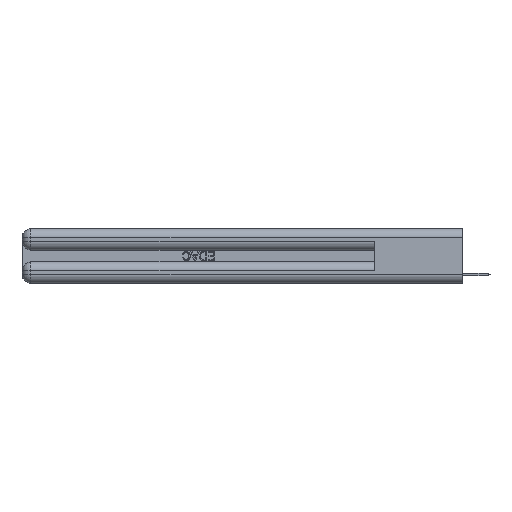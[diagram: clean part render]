
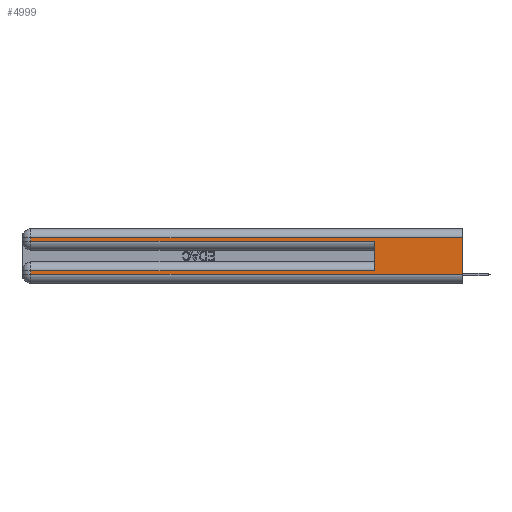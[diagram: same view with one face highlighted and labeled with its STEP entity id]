
A CAD part, left-side view. The second image highlights one B-rep face of the part: STEP entity #4999.
In plain terms, the highlighted planar face has unit normal (-1, 0, 0).
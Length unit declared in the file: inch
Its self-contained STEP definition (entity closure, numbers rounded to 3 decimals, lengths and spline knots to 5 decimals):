
#286 = EDGE_CURVE ( 'NONE', #21872, #2291, #27321, .T. ) ;
#1139 = CARTESIAN_POINT ( 'NONE',  ( 0., 0.6, 0.145 ) ) ;
#1155 = VECTOR ( 'NONE', #3932, 39.37008 ) ;
#2291 = VERTEX_POINT ( 'NONE', #21210 ) ;
#3072 = CARTESIAN_POINT ( 'NONE',  ( 0., 2.94, 0.06 ) ) ;
#3932 = DIRECTION ( 'NONE',  ( 0., -1., 0. ) ) ;
#4457 = FACE_OUTER_BOUND ( 'NONE', #8064, .T. ) ;
#4999 = ADVANCED_FACE ( 'NONE', ( #4457 ), #14202, .F. ) ;
#5020 = LINE ( 'NONE', #7411, #5801 ) ;
#5404 = VERTEX_POINT ( 'NONE', #13728 ) ;
#5482 = ORIENTED_EDGE ( 'NONE', *, *, #11655, .T. ) ;
#5722 = CARTESIAN_POINT ( 'NONE',  ( 0., 2.94, 0.285 ) ) ;
#5801 = VECTOR ( 'NONE', #27592, 39.37008 ) ;
#5935 = VECTOR ( 'NONE', #7160, 39.37008 ) ;
#6529 = ORIENTED_EDGE ( 'NONE', *, *, #286, .T. ) ;
#6652 = VERTEX_POINT ( 'NONE', #5722 ) ;
#7160 = DIRECTION ( 'NONE',  ( 0., 0., -1. ) ) ;
#7411 = CARTESIAN_POINT ( 'NONE',  ( 0., 0., 0.37 ) ) ;
#7462 = VECTOR ( 'NONE', #11444, 39.37008 ) ;
#7472 = VERTEX_POINT ( 'NONE', #28420 ) ;
#8064 = EDGE_LOOP ( 'NONE', ( #13339, #16782, #17089, #28735, #31666, #5482, #27351, #6529 ) ) ;
#8271 = EDGE_CURVE ( 'NONE', #6652, #22296, #17058, .T. ) ;
#9821 = CARTESIAN_POINT ( 'NONE',  ( 0., 0.6, 0.285 ) ) ;
#10339 = LINE ( 'NONE', #24592, #5935 ) ;
#11444 = DIRECTION ( 'NONE',  ( 0., 0., -1. ) ) ;
#11655 = EDGE_CURVE ( 'NONE', #20046, #5404, #31881, .T. ) ;
#12209 = LINE ( 'NONE', #31025, #7462 ) ;
#13339 = ORIENTED_EDGE ( 'NONE', *, *, #27402, .F. ) ;
#13593 = DIRECTION ( 'NONE',  ( 1., 0., 0. ) ) ;
#13728 = CARTESIAN_POINT ( 'NONE',  ( 0., 2.94, 0.085 ) ) ;
#13977 = CARTESIAN_POINT ( 'NONE',  ( 0., 0., 0.06 ) ) ;
#14202 = PLANE ( 'NONE',  #23083 ) ;
#15010 = EDGE_CURVE ( 'NONE', #5404, #21872, #12209, .T. ) ;
#16782 = ORIENTED_EDGE ( 'NONE', *, *, #26532, .T. ) ;
#17058 = LINE ( 'NONE', #18212, #17872 ) ;
#17089 = ORIENTED_EDGE ( 'NONE', *, *, #31121, .T. ) ;
#17872 = VECTOR ( 'NONE', #28212, 39.37008 ) ;
#18212 = CARTESIAN_POINT ( 'NONE',  ( 0., 0., 0.285 ) ) ;
#18639 = CARTESIAN_POINT ( 'NONE',  ( 0., 0., 0.31 ) ) ;
#20046 = VERTEX_POINT ( 'NONE', #26240 ) ;
#21210 = CARTESIAN_POINT ( 'NONE',  ( 0., 0., 0.06 ) ) ;
#21403 = DIRECTION ( 'NONE',  ( 0., 0., 1. ) ) ;
#21468 = EDGE_CURVE ( 'NONE', #20046, #22296, #30388, .T. ) ;
#21872 = VERTEX_POINT ( 'NONE', #3072 ) ;
#22296 = VERTEX_POINT ( 'NONE', #9821 ) ;
#23083 = AXIS2_PLACEMENT_3D ( 'NONE', #27799, #13593, #30604 ) ;
#23986 = VERTEX_POINT ( 'NONE', #25647 ) ;
#24088 = VECTOR ( 'NONE', #31932, 39.37008 ) ;
#24592 = CARTESIAN_POINT ( 'NONE',  ( 0., 2.94, 0.37 ) ) ;
#25647 = CARTESIAN_POINT ( 'NONE',  ( 0., 0., 0.31 ) ) ;
#26240 = CARTESIAN_POINT ( 'NONE',  ( 0., 0.6, 0.085 ) ) ;
#26532 = EDGE_CURVE ( 'NONE', #23986, #7472, #30804, .T. ) ;
#26817 = VECTOR ( 'NONE', #21403, 39.37008 ) ;
#27321 = LINE ( 'NONE', #13977, #1155 ) ;
#27351 = ORIENTED_EDGE ( 'NONE', *, *, #15010, .T. ) ;
#27402 = EDGE_CURVE ( 'NONE', #23986, #2291, #5020, .T. ) ;
#27592 = DIRECTION ( 'NONE',  ( 0., 0., -1. ) ) ;
#27799 = CARTESIAN_POINT ( 'NONE',  ( 0., 0., 0.37 ) ) ;
#27814 = CARTESIAN_POINT ( 'NONE',  ( 0., 0., 0.085 ) ) ;
#28212 = DIRECTION ( 'NONE',  ( 0., -1., 0. ) ) ;
#28246 = DIRECTION ( 'NONE',  ( 0., 1., 0. ) ) ;
#28420 = CARTESIAN_POINT ( 'NONE',  ( 0., 2.94, 0.31 ) ) ;
#28735 = ORIENTED_EDGE ( 'NONE', *, *, #8271, .T. ) ;
#30388 = LINE ( 'NONE', #1139, #26817 ) ;
#30604 = DIRECTION ( 'NONE',  ( 0., 0., -1. ) ) ;
#30680 = VECTOR ( 'NONE', #28246, 39.37008 ) ;
#30804 = LINE ( 'NONE', #18639, #24088 ) ;
#31025 = CARTESIAN_POINT ( 'NONE',  ( 0., 2.94, 0.37 ) ) ;
#31121 = EDGE_CURVE ( 'NONE', #7472, #6652, #10339, .T. ) ;
#31666 = ORIENTED_EDGE ( 'NONE', *, *, #21468, .F. ) ;
#31881 = LINE ( 'NONE', #27814, #30680 ) ;
#31932 = DIRECTION ( 'NONE',  ( 0., 1., 0. ) ) ;
